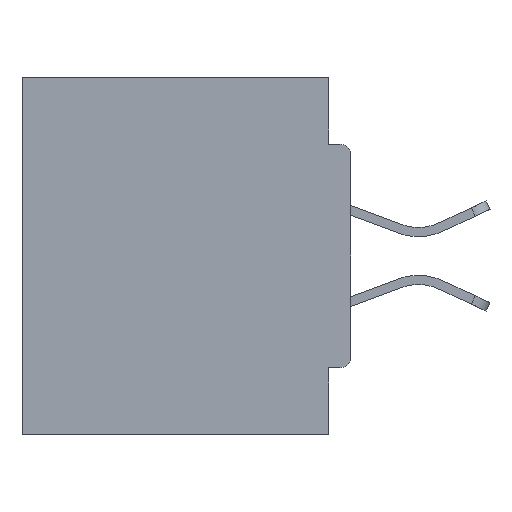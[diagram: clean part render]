
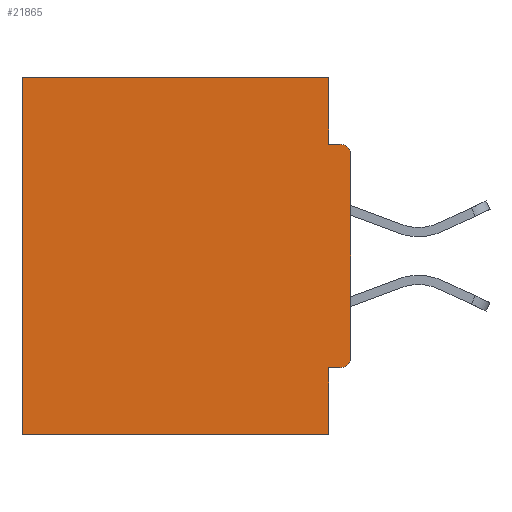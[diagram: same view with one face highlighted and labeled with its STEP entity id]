
A CAD part, left-side view. The second image highlights one B-rep face of the part: STEP entity #21865.
In plain terms, the highlighted planar face has unit normal (-1, 0, 0).
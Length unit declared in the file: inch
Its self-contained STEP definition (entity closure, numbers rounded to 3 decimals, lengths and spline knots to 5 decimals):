
#154 = CARTESIAN_POINT ( 'NONE',  ( 0.298, 0., 0. ) ) ;
#442 = ORIENTED_EDGE ( 'NONE', *, *, #34714, .T. ) ;
#443 = LINE ( 'NONE', #10744, #34203 ) ;
#2057 = VERTEX_POINT ( 'NONE', #28639 ) ;
#2212 = VECTOR ( 'NONE', #32360, 39.37008 ) ;
#2276 = DIRECTION ( 'NONE',  ( -1., 0., 0. ) ) ;
#2454 = VERTEX_POINT ( 'NONE', #9114 ) ;
#2762 = CARTESIAN_POINT ( 'NONE',  ( 0.298, 0., -0.1085 ) ) ;
#3563 = VERTEX_POINT ( 'NONE', #30096 ) ;
#3796 = VECTOR ( 'NONE', #9858, 39.37008 ) ;
#4642 = VECTOR ( 'NONE', #19846, 39.37008 ) ;
#4827 = CARTESIAN_POINT ( 'NONE',  ( 0.298, 0.015, -0.4065 ) ) ;
#4905 = ORIENTED_EDGE ( 'NONE', *, *, #22352, .T. ) ;
#5098 = CARTESIAN_POINT ( 'NONE',  ( 0.298, 0., -0.0935 ) ) ;
#5485 = AXIS2_PLACEMENT_3D ( 'NONE', #154, #11151, #8342 ) ;
#5797 = VECTOR ( 'NONE', #29078, 39.37008 ) ;
#6211 = VERTEX_POINT ( 'NONE', #2762 ) ;
#6844 = LINE ( 'NONE', #33588, #9486 ) ;
#7023 = CARTESIAN_POINT ( 'NONE',  ( 0.298, 0.46, 0. ) ) ;
#7043 = DIRECTION ( 'NONE',  ( 0., 0., -1. ) ) ;
#8342 = DIRECTION ( 'NONE',  ( 0., 0., -1. ) ) ;
#8458 = EDGE_CURVE ( 'NONE', #33398, #3563, #19979, .T. ) ;
#8623 = AXIS2_PLACEMENT_3D ( 'NONE', #10693, #2276, #22104 ) ;
#8749 = DIRECTION ( 'NONE',  ( 0., 0., -1. ) ) ;
#8858 = DIRECTION ( 'NONE',  ( -1., 0., 0. ) ) ;
#8899 = FACE_OUTER_BOUND ( 'NONE', #14468, .T. ) ;
#9114 = CARTESIAN_POINT ( 'NONE',  ( 0.298, 0., -0.3915 ) ) ;
#9226 = CARTESIAN_POINT ( 'NONE',  ( 0.298, 0.031, -0.5 ) ) ;
#9486 = VECTOR ( 'NONE', #8749, 39.37008 ) ;
#9580 = LINE ( 'NONE', #7023, #3796 ) ;
#9858 = DIRECTION ( 'NONE',  ( 0., 0., -1. ) ) ;
#10693 = CARTESIAN_POINT ( 'NONE',  ( 0.298, 0.015, -0.3915 ) ) ;
#10744 = CARTESIAN_POINT ( 'NONE',  ( 0.298, 0., 0. ) ) ;
#10867 = EDGE_CURVE ( 'NONE', #33474, #2057, #9580, .T. ) ;
#11151 = DIRECTION ( 'NONE',  ( 1., 0., 0. ) ) ;
#11218 = AXIS2_PLACEMENT_3D ( 'NONE', #11927, #8858, #31826 ) ;
#11389 = CARTESIAN_POINT ( 'NONE',  ( 0.298, 0.46, 0. ) ) ;
#11813 = LINE ( 'NONE', #20287, #30029 ) ;
#11927 = CARTESIAN_POINT ( 'NONE',  ( 0.298, 0.015, -0.1085 ) ) ;
#12964 = ORIENTED_EDGE ( 'NONE', *, *, #30308, .F. ) ;
#14468 = EDGE_LOOP ( 'NONE', ( #22979, #12964, #30242, #4905, #30469, #24368, #14737, #29187, #442, #36047 ) ) ;
#14737 = ORIENTED_EDGE ( 'NONE', *, *, #32208, .F. ) ;
#15196 = VECTOR ( 'NONE', #24954, 39.37008 ) ;
#15496 = CARTESIAN_POINT ( 'NONE',  ( 0.298, 0.031, -0.0935 ) ) ;
#16752 = CARTESIAN_POINT ( 'NONE',  ( 0.298, 0., -0.5 ) ) ;
#17400 = CARTESIAN_POINT ( 'NONE',  ( 0.298, 0.015, -0.0935 ) ) ;
#19301 = DIRECTION ( 'NONE',  ( 0., 1., 0. ) ) ;
#19846 = DIRECTION ( 'NONE',  ( 0., 1., 0. ) ) ;
#19889 = EDGE_CURVE ( 'NONE', #6211, #2454, #6844, .T. ) ;
#19979 = LINE ( 'NONE', #32497, #2212 ) ;
#20287 = CARTESIAN_POINT ( 'NONE',  ( 0.298, 0.031, -0.5 ) ) ;
#21487 = EDGE_CURVE ( 'NONE', #24758, #31469, #25355, .T. ) ;
#21865 = ADVANCED_FACE ( 'NONE', ( #8899 ), #25579, .F. ) ;
#22104 = DIRECTION ( 'NONE',  ( 0., 0., -1. ) ) ;
#22352 = EDGE_CURVE ( 'NONE', #24758, #33474, #443, .T. ) ;
#22979 = ORIENTED_EDGE ( 'NONE', *, *, #24231, .T. ) ;
#24231 = EDGE_CURVE ( 'NONE', #6211, #27674, #32228, .T. ) ;
#24368 = ORIENTED_EDGE ( 'NONE', *, *, #28784, .F. ) ;
#24758 = VERTEX_POINT ( 'NONE', #31566 ) ;
#24954 = DIRECTION ( 'NONE',  ( 0., -1., 0. ) ) ;
#25355 = LINE ( 'NONE', #9226, #5797 ) ;
#25579 = PLANE ( 'NONE',  #5485 ) ;
#27609 = LINE ( 'NONE', #5098, #15196 ) ;
#27674 = VERTEX_POINT ( 'NONE', #17400 ) ;
#28639 = CARTESIAN_POINT ( 'NONE',  ( 0.298, 0.46, -0.5 ) ) ;
#28784 = EDGE_CURVE ( 'NONE', #31876, #2057, #29977, .T. ) ;
#29078 = DIRECTION ( 'NONE',  ( 0., 0., -1. ) ) ;
#29187 = ORIENTED_EDGE ( 'NONE', *, *, #8458, .F. ) ;
#29977 = LINE ( 'NONE', #16752, #4642 ) ;
#30029 = VECTOR ( 'NONE', #7043, 39.37008 ) ;
#30096 = CARTESIAN_POINT ( 'NONE',  ( 0.298, 0.031, -0.4065 ) ) ;
#30242 = ORIENTED_EDGE ( 'NONE', *, *, #21487, .F. ) ;
#30308 = EDGE_CURVE ( 'NONE', #31469, #27674, #27609, .T. ) ;
#30469 = ORIENTED_EDGE ( 'NONE', *, *, #10867, .T. ) ;
#31469 = VERTEX_POINT ( 'NONE', #15496 ) ;
#31566 = CARTESIAN_POINT ( 'NONE',  ( 0.298, 0.031, 0. ) ) ;
#31826 = DIRECTION ( 'NONE',  ( 0., 0., -1. ) ) ;
#31876 = VERTEX_POINT ( 'NONE', #34366 ) ;
#32208 = EDGE_CURVE ( 'NONE', #3563, #31876, #11813, .T. ) ;
#32228 = CIRCLE ( 'NONE', #11218, 0.015 ) ;
#32360 = DIRECTION ( 'NONE',  ( 0., 1., 0. ) ) ;
#32497 = CARTESIAN_POINT ( 'NONE',  ( 0.298, 0., -0.4065 ) ) ;
#33398 = VERTEX_POINT ( 'NONE', #4827 ) ;
#33474 = VERTEX_POINT ( 'NONE', #11389 ) ;
#33588 = CARTESIAN_POINT ( 'NONE',  ( 0.298, 0., 0. ) ) ;
#34203 = VECTOR ( 'NONE', #19301, 39.37008 ) ;
#34366 = CARTESIAN_POINT ( 'NONE',  ( 0.298, 0.031, -0.5 ) ) ;
#34714 = EDGE_CURVE ( 'NONE', #33398, #2454, #36151, .T. ) ;
#36047 = ORIENTED_EDGE ( 'NONE', *, *, #19889, .F. ) ;
#36151 = CIRCLE ( 'NONE', #8623, 0.015 ) ;
